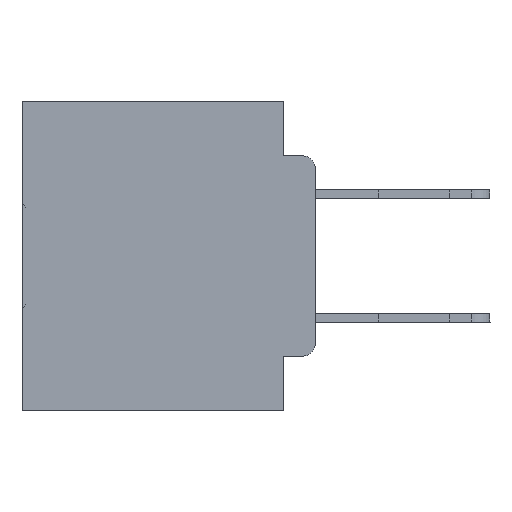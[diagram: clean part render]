
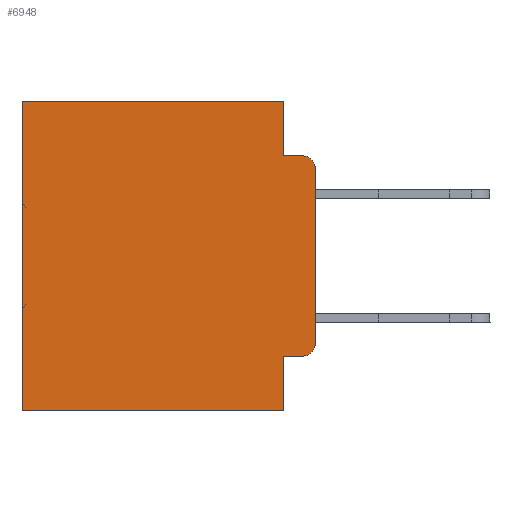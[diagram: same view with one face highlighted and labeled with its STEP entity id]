
A CAD part, left-side view. The second image highlights one B-rep face of the part: STEP entity #6948.
In plain terms, the highlighted planar face has unit normal (-1, 0, 0).
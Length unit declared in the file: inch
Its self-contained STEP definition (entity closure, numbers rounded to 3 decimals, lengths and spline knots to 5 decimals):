
#97 = VECTOR ( 'NONE', #13814, 39.37008 ) ;
#322 = LINE ( 'NONE', #18738, #97 ) ;
#388 = AXIS2_PLACEMENT_3D ( 'NONE', #5092, #15811, #9936 ) ;
#451 = CARTESIAN_POINT ( 'NONE',  ( 0.298, 0., -0.5 ) ) ;
#722 = VECTOR ( 'NONE', #18086, 39.37008 ) ;
#887 = LINE ( 'NONE', #11565, #27486 ) ;
#972 = CARTESIAN_POINT ( 'NONE',  ( 0.298, 0.02, -0.3915 ) ) ;
#1092 = EDGE_LOOP ( 'NONE', ( #12380, #3949, #24712, #16365, #23433, #24517, #8681, #5463, #33676, #23072 ) ) ;
#2176 = VERTEX_POINT ( 'NONE', #27096 ) ;
#2209 = DIRECTION ( 'NONE',  ( 0., -1., 0. ) ) ;
#2370 = VERTEX_POINT ( 'NONE', #3838 ) ;
#2928 = CARTESIAN_POINT ( 'NONE',  ( 0.298, 0., 0. ) ) ;
#3103 = LINE ( 'NONE', #32683, #25645 ) ;
#3304 = EDGE_CURVE ( 'NONE', #15544, #14780, #16104, .T. ) ;
#3838 = CARTESIAN_POINT ( 'NONE',  ( 0.298, 0., -0.1085 ) ) ;
#3839 = CARTESIAN_POINT ( 'NONE',  ( 0.298, 0.051, -0.5 ) ) ;
#3923 = EDGE_CURVE ( 'NONE', #19265, #2176, #5212, .T. ) ;
#3949 = ORIENTED_EDGE ( 'NONE', *, *, #9454, .T. ) ;
#5092 = CARTESIAN_POINT ( 'NONE',  ( 0.298, 0., 0. ) ) ;
#5212 = CIRCLE ( 'NONE', #22654, 0.02 ) ;
#5463 = ORIENTED_EDGE ( 'NONE', *, *, #23129, .F. ) ;
#6209 = LINE ( 'NONE', #451, #15201 ) ;
#6418 = CARTESIAN_POINT ( 'NONE',  ( 0.298, 0.051, 0. ) ) ;
#6706 = EDGE_CURVE ( 'NONE', #2370, #2176, #3103, .T. ) ;
#6803 = VERTEX_POINT ( 'NONE', #6418 ) ;
#6948 = ADVANCED_FACE ( 'NONE', ( #15634 ), #26421, .F. ) ;
#7735 = EDGE_CURVE ( 'NONE', #11415, #19265, #26318, .T. ) ;
#8681 = ORIENTED_EDGE ( 'NONE', *, *, #32501, .F. ) ;
#9454 = EDGE_CURVE ( 'NONE', #2370, #21735, #21745, .T. ) ;
#9936 = DIRECTION ( 'NONE',  ( 0., 0., -1. ) ) ;
#10552 = VERTEX_POINT ( 'NONE', #3839 ) ;
#11415 = VERTEX_POINT ( 'NONE', #13431 ) ;
#11565 = CARTESIAN_POINT ( 'NONE',  ( 0.298, 0.051, -0.0885 ) ) ;
#11652 = DIRECTION ( 'NONE',  ( -1., 0., 0. ) ) ;
#11678 = LINE ( 'NONE', #2928, #31278 ) ;
#12380 = ORIENTED_EDGE ( 'NONE', *, *, #6706, .F. ) ;
#13431 = CARTESIAN_POINT ( 'NONE',  ( 0.298, 0.051, -0.4115 ) ) ;
#13642 = DIRECTION ( 'NONE',  ( 0., 0., -1. ) ) ;
#13814 = DIRECTION ( 'NONE',  ( 0., 0., -1. ) ) ;
#14780 = VERTEX_POINT ( 'NONE', #34237 ) ;
#15060 = CARTESIAN_POINT ( 'NONE',  ( 0.298, 0.02, -0.4115 ) ) ;
#15201 = VECTOR ( 'NONE', #27546, 39.37008 ) ;
#15544 = VERTEX_POINT ( 'NONE', #30278 ) ;
#15634 = FACE_OUTER_BOUND ( 'NONE', #1092, .T. ) ;
#15811 = DIRECTION ( 'NONE',  ( 1., 0., 0. ) ) ;
#16104 = LINE ( 'NONE', #21926, #27128 ) ;
#16365 = ORIENTED_EDGE ( 'NONE', *, *, #33774, .F. ) ;
#17561 = CARTESIAN_POINT ( 'NONE',  ( 0.298, 0.02, -0.0885 ) ) ;
#17628 = DIRECTION ( 'NONE',  ( 0., 0., -1. ) ) ;
#18086 = DIRECTION ( 'NONE',  ( 0., 0., -1. ) ) ;
#18738 = CARTESIAN_POINT ( 'NONE',  ( 0.298, 0.051, 0. ) ) ;
#19162 = VERTEX_POINT ( 'NONE', #27252 ) ;
#19265 = VERTEX_POINT ( 'NONE', #15060 ) ;
#19794 = DIRECTION ( 'NONE',  ( 0., 1., 0. ) ) ;
#21735 = VERTEX_POINT ( 'NONE', #17561 ) ;
#21745 = CIRCLE ( 'NONE', #24582, 0.02 ) ;
#21926 = CARTESIAN_POINT ( 'NONE',  ( 0.298, 0.473, 0. ) ) ;
#22654 = AXIS2_PLACEMENT_3D ( 'NONE', #972, #11652, #30696 ) ;
#23072 = ORIENTED_EDGE ( 'NONE', *, *, #3923, .T. ) ;
#23129 = EDGE_CURVE ( 'NONE', #11415, #10552, #29399, .T. ) ;
#23433 = ORIENTED_EDGE ( 'NONE', *, *, #26674, .T. ) ;
#24019 = VECTOR ( 'NONE', #2209, 39.37008 ) ;
#24517 = ORIENTED_EDGE ( 'NONE', *, *, #3304, .T. ) ;
#24582 = AXIS2_PLACEMENT_3D ( 'NONE', #33899, #31060, #17628 ) ;
#24712 = ORIENTED_EDGE ( 'NONE', *, *, #30126, .F. ) ;
#25645 = VECTOR ( 'NONE', #30019, 39.37008 ) ;
#26318 = LINE ( 'NONE', #28939, #24019 ) ;
#26421 = PLANE ( 'NONE',  #388 ) ;
#26674 = EDGE_CURVE ( 'NONE', #6803, #15544, #11678, .T. ) ;
#27096 = CARTESIAN_POINT ( 'NONE',  ( 0.298, 0., -0.3915 ) ) ;
#27128 = VECTOR ( 'NONE', #13642, 39.37008 ) ;
#27252 = CARTESIAN_POINT ( 'NONE',  ( 0.298, 0.051, -0.0885 ) ) ;
#27486 = VECTOR ( 'NONE', #32908, 39.37008 ) ;
#27546 = DIRECTION ( 'NONE',  ( 0., 1., 0. ) ) ;
#28939 = CARTESIAN_POINT ( 'NONE',  ( 0.298, 0.051, -0.4115 ) ) ;
#29399 = LINE ( 'NONE', #34356, #722 ) ;
#30019 = DIRECTION ( 'NONE',  ( 0., 0., -1. ) ) ;
#30126 = EDGE_CURVE ( 'NONE', #19162, #21735, #887, .T. ) ;
#30278 = CARTESIAN_POINT ( 'NONE',  ( 0.298, 0.473, 0. ) ) ;
#30696 = DIRECTION ( 'NONE',  ( 0., 0., -1. ) ) ;
#31060 = DIRECTION ( 'NONE',  ( -1., 0., 0. ) ) ;
#31278 = VECTOR ( 'NONE', #19794, 39.37008 ) ;
#32501 = EDGE_CURVE ( 'NONE', #10552, #14780, #6209, .T. ) ;
#32683 = CARTESIAN_POINT ( 'NONE',  ( 0.298, 0., 0. ) ) ;
#32908 = DIRECTION ( 'NONE',  ( 0., -1., 0. ) ) ;
#33676 = ORIENTED_EDGE ( 'NONE', *, *, #7735, .T. ) ;
#33774 = EDGE_CURVE ( 'NONE', #6803, #19162, #322, .T. ) ;
#33899 = CARTESIAN_POINT ( 'NONE',  ( 0.298, 0.02, -0.1085 ) ) ;
#34237 = CARTESIAN_POINT ( 'NONE',  ( 0.298, 0.473, -0.5 ) ) ;
#34356 = CARTESIAN_POINT ( 'NONE',  ( 0.298, 0.051, 0. ) ) ;
